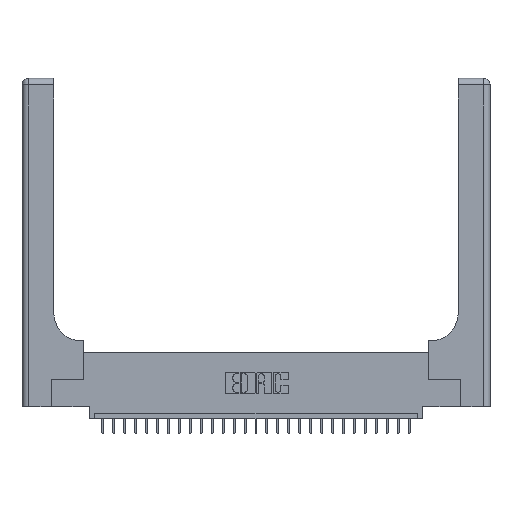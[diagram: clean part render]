
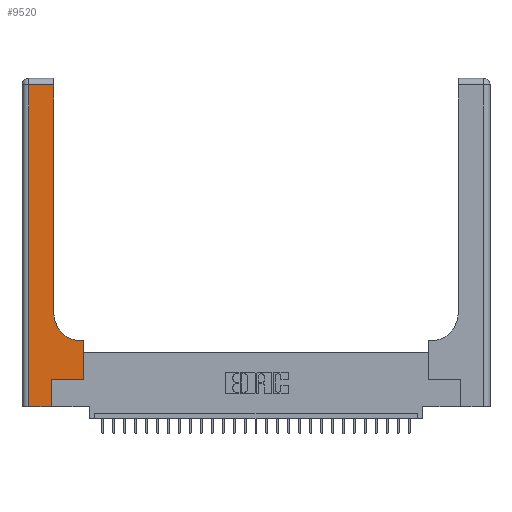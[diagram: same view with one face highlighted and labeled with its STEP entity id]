
A CAD part, top view. The second image highlights one B-rep face of the part: STEP entity #9520.
In plain terms, the highlighted planar face has unit normal (0, 0, 1).
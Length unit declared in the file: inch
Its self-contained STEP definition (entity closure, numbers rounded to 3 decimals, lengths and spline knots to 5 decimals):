
#602 = DIRECTION ( 'NONE',  ( 0., 1., 0. ) ) ;
#638 = PLANE ( 'NONE',  #21060 ) ;
#712 = CARTESIAN_POINT ( 'NONE',  ( 0.269, 0., 0.37 ) ) ;
#1925 = VECTOR ( 'NONE', #26682, 39.37008 ) ;
#1935 = VERTEX_POINT ( 'NONE', #14019 ) ;
#1967 = CARTESIAN_POINT ( 'NONE',  ( 0., 2.94, 0.37 ) ) ;
#2267 = CARTESIAN_POINT ( 'NONE',  ( 0., 0., 0.37 ) ) ;
#3305 = VERTEX_POINT ( 'NONE', #5567 ) ;
#3346 = EDGE_LOOP ( 'NONE', ( #23534, #27166, #22593, #8879, #21366, #12433, #22240, #13318, #23610 ) ) ;
#4487 = EDGE_CURVE ( 'NONE', #25665, #10976, #16748, .T. ) ;
#4782 = FACE_OUTER_BOUND ( 'NONE', #3346, .T. ) ;
#5567 = CARTESIAN_POINT ( 'NONE',  ( 0.5585, 0.25, 0.37 ) ) ;
#5632 = EDGE_CURVE ( 'NONE', #26489, #7812, #22303, .T. ) ;
#5660 = EDGE_CURVE ( 'NONE', #18717, #25665, #22797, .T. ) ;
#5697 = DIRECTION ( 'NONE',  ( -1., 0., 0. ) ) ;
#6220 = CARTESIAN_POINT ( 'NONE',  ( 0.269, 0.25, 0.37 ) ) ;
#6977 = DIRECTION ( 'NONE',  ( -1., 0., 0. ) ) ;
#7812 = VERTEX_POINT ( 'NONE', #18724 ) ;
#8282 = EDGE_CURVE ( 'NONE', #1935, #26489, #18546, .T. ) ;
#8430 = CARTESIAN_POINT ( 'NONE',  ( 0.269, 0.25, 0.37 ) ) ;
#8470 = DIRECTION ( 'NONE',  ( 1., 0., 0. ) ) ;
#8879 = ORIENTED_EDGE ( 'NONE', *, *, #5660, .T. ) ;
#9331 = DIRECTION ( 'NONE',  ( -1., 0., 0. ) ) ;
#9471 = EDGE_CURVE ( 'NONE', #9505, #21986, #22065, .T. ) ;
#9505 = VERTEX_POINT ( 'NONE', #27054 ) ;
#9520 = ADVANCED_FACE ( 'NONE', ( #4782 ), #638, .F. ) ;
#9994 = EDGE_CURVE ( 'NONE', #7812, #9505, #27466, .T. ) ;
#10665 = VECTOR ( 'NONE', #25257, 39.37008 ) ;
#10681 = CARTESIAN_POINT ( 'NONE',  ( 0.5415, 0.85, 0.37 ) ) ;
#10976 = VERTEX_POINT ( 'NONE', #6220 ) ;
#11513 = CARTESIAN_POINT ( 'NONE',  ( 0.06, 0., 0.37 ) ) ;
#11660 = CARTESIAN_POINT ( 'NONE',  ( 0.5415, 0.6, 0.37 ) ) ;
#12433 = ORIENTED_EDGE ( 'NONE', *, *, #23096, .T. ) ;
#12904 = VECTOR ( 'NONE', #19642, 39.37008 ) ;
#13318 = ORIENTED_EDGE ( 'NONE', *, *, #8282, .T. ) ;
#14019 = CARTESIAN_POINT ( 'NONE',  ( 0.5585, 0.6, 0.37 ) ) ;
#14560 = VECTOR ( 'NONE', #9331, 39.37008 ) ;
#15336 = AXIS2_PLACEMENT_3D ( 'NONE', #10681, #28550, #8470 ) ;
#15416 = LINE ( 'NONE', #26247, #12904 ) ;
#16320 = CARTESIAN_POINT ( 'NONE',  ( 0.269, 0., 0.37 ) ) ;
#16485 = VECTOR ( 'NONE', #17314, 39.37008 ) ;
#16748 = LINE ( 'NONE', #16320, #10665 ) ;
#17314 = DIRECTION ( 'NONE',  ( 0., 1., 0. ) ) ;
#17347 = LINE ( 'NONE', #8430, #1925 ) ;
#17369 = VECTOR ( 'NONE', #602, 39.37008 ) ;
#17749 = LINE ( 'NONE', #21863, #16485 ) ;
#18087 = DIRECTION ( 'NONE',  ( 0., 0., -1. ) ) ;
#18109 = VECTOR ( 'NONE', #24415, 39.37008 ) ;
#18546 = LINE ( 'NONE', #23259, #21952 ) ;
#18717 = VERTEX_POINT ( 'NONE', #11513 ) ;
#18724 = CARTESIAN_POINT ( 'NONE',  ( 0.2915, 0.85, 0.37 ) ) ;
#19642 = DIRECTION ( 'NONE',  ( 0., -1., 0. ) ) ;
#20254 = CARTESIAN_POINT ( 'NONE',  ( 0.2915, 3., 0.37 ) ) ;
#21060 = AXIS2_PLACEMENT_3D ( 'NONE', #23067, #18087, #6977 ) ;
#21366 = ORIENTED_EDGE ( 'NONE', *, *, #4487, .T. ) ;
#21863 = CARTESIAN_POINT ( 'NONE',  ( 0.5585, 0.25, 0.37 ) ) ;
#21952 = VECTOR ( 'NONE', #5697, 39.37008 ) ;
#21986 = VERTEX_POINT ( 'NONE', #26089 ) ;
#22065 = LINE ( 'NONE', #1967, #14560 ) ;
#22240 = ORIENTED_EDGE ( 'NONE', *, *, #28473, .T. ) ;
#22303 = CIRCLE ( 'NONE', #15336, 0.25 ) ;
#22593 = ORIENTED_EDGE ( 'NONE', *, *, #27237, .T. ) ;
#22797 = LINE ( 'NONE', #2267, #18109 ) ;
#23067 = CARTESIAN_POINT ( 'NONE',  ( 0., 3., 0.37 ) ) ;
#23096 = EDGE_CURVE ( 'NONE', #10976, #3305, #17347, .T. ) ;
#23259 = CARTESIAN_POINT ( 'NONE',  ( 0.2915, 0.6, 0.37 ) ) ;
#23534 = ORIENTED_EDGE ( 'NONE', *, *, #9994, .T. ) ;
#23610 = ORIENTED_EDGE ( 'NONE', *, *, #5632, .T. ) ;
#24415 = DIRECTION ( 'NONE',  ( 1., 0., 0. ) ) ;
#25257 = DIRECTION ( 'NONE',  ( 0., 1., 0. ) ) ;
#25665 = VERTEX_POINT ( 'NONE', #712 ) ;
#26089 = CARTESIAN_POINT ( 'NONE',  ( 0.06, 2.94, 0.37 ) ) ;
#26247 = CARTESIAN_POINT ( 'NONE',  ( 0.06, 3., 0.37 ) ) ;
#26489 = VERTEX_POINT ( 'NONE', #11660 ) ;
#26682 = DIRECTION ( 'NONE',  ( 1., 0., 0. ) ) ;
#27054 = CARTESIAN_POINT ( 'NONE',  ( 0.2915, 2.94, 0.37 ) ) ;
#27166 = ORIENTED_EDGE ( 'NONE', *, *, #9471, .T. ) ;
#27237 = EDGE_CURVE ( 'NONE', #21986, #18717, #15416, .T. ) ;
#27466 = LINE ( 'NONE', #20254, #17369 ) ;
#28473 = EDGE_CURVE ( 'NONE', #3305, #1935, #17749, .T. ) ;
#28550 = DIRECTION ( 'NONE',  ( 0., 0., -1. ) ) ;
